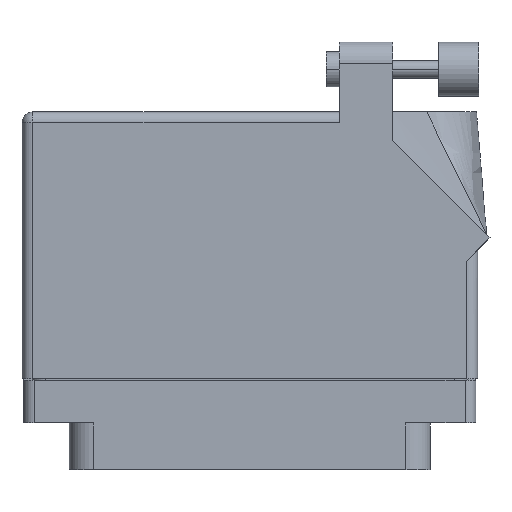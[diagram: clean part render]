
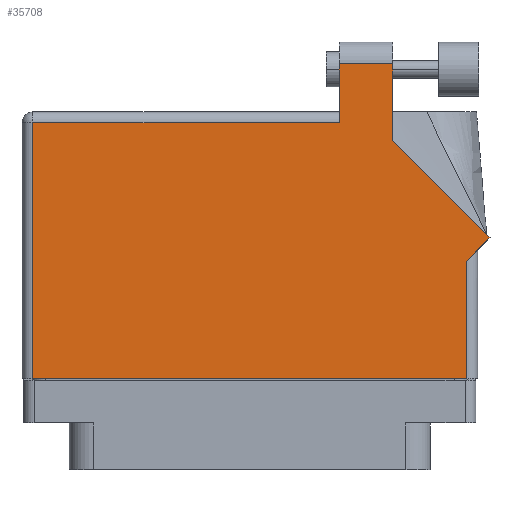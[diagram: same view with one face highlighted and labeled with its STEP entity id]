
A CAD part, front view. The second image highlights one B-rep face of the part: STEP entity #35708.
In plain terms, the highlighted face is planar.
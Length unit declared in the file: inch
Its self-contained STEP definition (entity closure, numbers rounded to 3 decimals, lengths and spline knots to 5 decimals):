
#1002 = CARTESIAN_POINT ( 'NONE',  ( -1.306, -0.1, 0.455 ) ) ;
#1747 = CARTESIAN_POINT ( 'NONE',  ( -1.244, -0.1, 0.455 ) ) ;
#1906 = CARTESIAN_POINT ( 'NONE',  ( 0.513, 1.705, 0.455 ) ) ;
#2969 = EDGE_CURVE ( 'NONE', #14198, #29208, #28104, .T. ) ;
#3308 = ORIENTED_EDGE ( 'NONE', *, *, #37932, .T. ) ;
#4177 = EDGE_CURVE ( 'NONE', #37669, #5509, #34416, .T. ) ;
#5509 = VERTEX_POINT ( 'NONE', #26759 ) ;
#5792 = VECTOR ( 'NONE', #46822, 39.37008 ) ;
#6041 = CARTESIAN_POINT ( 'NONE',  ( 0.82, 1.705, 0.455 ) ) ;
#6305 = LINE ( 'NONE', #10158, #18370 ) ;
#7761 = LINE ( 'NONE', #34140, #34067 ) ;
#8790 = LINE ( 'NONE', #19945, #13475 ) ;
#9509 = EDGE_CURVE ( 'NONE', #28134, #37756, #32415, .T. ) ;
#10158 = CARTESIAN_POINT ( 'NONE',  ( -1.244, -0.1, 0.455 ) ) ;
#10395 = DIRECTION ( 'NONE',  ( -1., 0., 0. ) ) ;
#10741 = VECTOR ( 'NONE', #14222, 39.37008 ) ;
#11983 = VECTOR ( 'NONE', #16484, 39.37008 ) ;
#13142 = FACE_OUTER_BOUND ( 'NONE', #19471, .T. ) ;
#13475 = VECTOR ( 'NONE', #34714, 39.37008 ) ;
#14198 = VERTEX_POINT ( 'NONE', #32334 ) ;
#14222 = DIRECTION ( 'NONE',  ( -0.707, 0.707, 0. ) ) ;
#14766 = ORIENTED_EDGE ( 'NONE', *, *, #39415, .T. ) ;
#15565 = VECTOR ( 'NONE', #35318, 39.37008 ) ;
#16484 = DIRECTION ( 'NONE',  ( 1., 0., 0. ) ) ;
#17282 = ORIENTED_EDGE ( 'NONE', *, *, #4177, .T. ) ;
#17381 = LINE ( 'NONE', #1906, #15565 ) ;
#17864 = CARTESIAN_POINT ( 'NONE',  ( 1.37671, 0.70771, 0.455 ) ) ;
#18370 = VECTOR ( 'NONE', #25665, 39.37008 ) ;
#18887 = DIRECTION ( 'NONE',  ( 0., 1., 0. ) ) ;
#19471 = EDGE_LOOP ( 'NONE', ( #21851, #36287, #29324, #20485, #39870, #17282, #3308, #14766, #44333 ) ) ;
#19945 = CARTESIAN_POINT ( 'NONE',  ( 0.82, 1.26442, 0.455 ) ) ;
#20458 = CARTESIAN_POINT ( 'NONE',  ( -1.244, 1.368, 0.455 ) ) ;
#20485 = ORIENTED_EDGE ( 'NONE', *, *, #2969, .T. ) ;
#21138 = CARTESIAN_POINT ( 'NONE',  ( -1.306, 1.43, 0.455 ) ) ;
#21546 = CARTESIAN_POINT ( 'NONE',  ( 0.513, 1.705, 0.455 ) ) ;
#21851 = ORIENTED_EDGE ( 'NONE', *, *, #26589, .T. ) ;
#25665 = DIRECTION ( 'NONE',  ( 0., -1., 0. ) ) ;
#25750 = LINE ( 'NONE', #33025, #5792 ) ;
#25875 = VECTOR ( 'NONE', #10395, 39.37008 ) ;
#26589 = EDGE_CURVE ( 'NONE', #37756, #36977, #8790, .T. ) ;
#26759 = CARTESIAN_POINT ( 'NONE',  ( 1.244, -0.1, 0.455 ) ) ;
#28104 = LINE ( 'NONE', #29075, #25875 ) ;
#28134 = VERTEX_POINT ( 'NONE', #43641 ) ;
#28173 = PLANE ( 'NONE',  #41899 ) ;
#28568 = VERTEX_POINT ( 'NONE', #21546 ) ;
#29075 = CARTESIAN_POINT ( 'NONE',  ( -1.306, 1.368, 0.455 ) ) ;
#29208 = VERTEX_POINT ( 'NONE', #20458 ) ;
#29324 = ORIENTED_EDGE ( 'NONE', *, *, #45324, .T. ) ;
#29688 = EDGE_CURVE ( 'NONE', #29208, #37669, #6305, .T. ) ;
#31217 = VERTEX_POINT ( 'NONE', #33240 ) ;
#32334 = CARTESIAN_POINT ( 'NONE',  ( 0.513, 1.368, 0.455 ) ) ;
#32415 = LINE ( 'NONE', #17864, #10741 ) ;
#33025 = CARTESIAN_POINT ( 'NONE',  ( 0.513, 1.43, 0.455 ) ) ;
#33240 = CARTESIAN_POINT ( 'NONE',  ( 1.244, 0.575, 0.455 ) ) ;
#34063 = VECTOR ( 'NONE', #46482, 39.37008 ) ;
#34067 = VECTOR ( 'NONE', #18887, 39.37008 ) ;
#34140 = CARTESIAN_POINT ( 'NONE',  ( 1.244, 0.637, 0.455 ) ) ;
#34416 = LINE ( 'NONE', #1002, #11983 ) ;
#34714 = DIRECTION ( 'NONE',  ( 0., 1., 0. ) ) ;
#35182 = DIRECTION ( 'NONE',  ( 0., 0., -1. ) ) ;
#35318 = DIRECTION ( 'NONE',  ( -1., 0., 0. ) ) ;
#35628 = CARTESIAN_POINT ( 'NONE',  ( 0.82, 1.26442, 0.455 ) ) ;
#35656 = DIRECTION ( 'NONE',  ( -1., 0., 0. ) ) ;
#35708 = ADVANCED_FACE ( 'NONE', ( #13142 ), #28173, .F. ) ;
#36287 = ORIENTED_EDGE ( 'NONE', *, *, #40319, .T. ) ;
#36977 = VERTEX_POINT ( 'NONE', #6041 ) ;
#37669 = VERTEX_POINT ( 'NONE', #1747 ) ;
#37756 = VERTEX_POINT ( 'NONE', #35628 ) ;
#37932 = EDGE_CURVE ( 'NONE', #5509, #31217, #7761, .T. ) ;
#39415 = EDGE_CURVE ( 'NONE', #31217, #28134, #45778, .T. ) ;
#39870 = ORIENTED_EDGE ( 'NONE', *, *, #29688, .T. ) ;
#40319 = EDGE_CURVE ( 'NONE', #36977, #28568, #17381, .T. ) ;
#41899 = AXIS2_PLACEMENT_3D ( 'NONE', #21138, #35182, #35656 ) ;
#43641 = CARTESIAN_POINT ( 'NONE',  ( 1.37671, 0.70771, 0.455 ) ) ;
#44333 = ORIENTED_EDGE ( 'NONE', *, *, #9509, .T. ) ;
#45324 = EDGE_CURVE ( 'NONE', #28568, #14198, #25750, .T. ) ;
#45778 = LINE ( 'NONE', #46722, #34063 ) ;
#46482 = DIRECTION ( 'NONE',  ( 0.707, 0.707, 0. ) ) ;
#46722 = CARTESIAN_POINT ( 'NONE',  ( 1.306, 0.637, 0.455 ) ) ;
#46822 = DIRECTION ( 'NONE',  ( 0., -1., 0. ) ) ;
